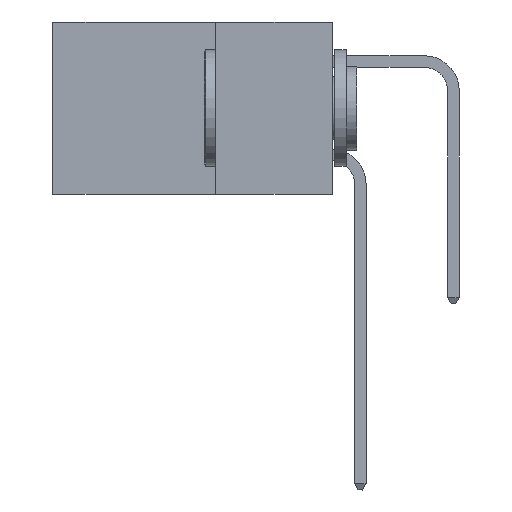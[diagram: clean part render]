
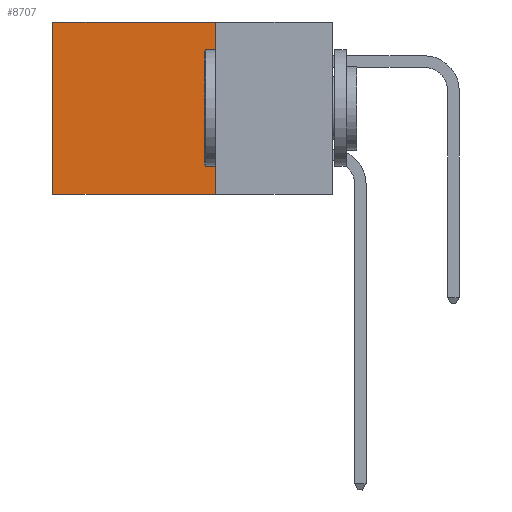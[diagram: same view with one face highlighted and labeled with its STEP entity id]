
A CAD part, left-side view. The second image highlights one B-rep face of the part: STEP entity #8707.
In plain terms, the highlighted planar face has unit normal (-1, 0, 0).
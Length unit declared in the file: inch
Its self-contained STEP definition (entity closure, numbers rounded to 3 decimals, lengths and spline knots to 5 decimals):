
#2173 = VERTEX_POINT ( 'NONE', #23005 ) ;
#2880 = LINE ( 'NONE', #3835, #20670 ) ;
#3231 = VERTEX_POINT ( 'NONE', #19657 ) ;
#3835 = CARTESIAN_POINT ( 'NONE',  ( 0.298, 0.25, 0. ) ) ;
#6220 = DIRECTION ( 'NONE',  ( 0., 0., -1. ) ) ;
#6695 = VECTOR ( 'NONE', #28479, 39.37008 ) ;
#6897 = CARTESIAN_POINT ( 'NONE',  ( 0.298, 0.6, -0.37 ) ) ;
#7433 = LINE ( 'NONE', #26157, #6695 ) ;
#7675 = ORIENTED_EDGE ( 'NONE', *, *, #19054, .T. ) ;
#8707 = ADVANCED_FACE ( 'NONE', ( #20876 ), #25672, .F. ) ;
#11441 = CARTESIAN_POINT ( 'NONE',  ( 0.298, 0.25, 0. ) ) ;
#13474 = EDGE_CURVE ( 'NONE', #2173, #17907, #7433, .T. ) ;
#13802 = DIRECTION ( 'NONE',  ( 0., 0., -1. ) ) ;
#14105 = EDGE_LOOP ( 'NONE', ( #31052, #15965, #26551, #7675 ) ) ;
#15561 = VECTOR ( 'NONE', #30053, 39.37008 ) ;
#15965 = ORIENTED_EDGE ( 'NONE', *, *, #29379, .F. ) ;
#15981 = VECTOR ( 'NONE', #29298, 39.37008 ) ;
#17104 = LINE ( 'NONE', #27704, #15561 ) ;
#17907 = VERTEX_POINT ( 'NONE', #6897 ) ;
#19054 = EDGE_CURVE ( 'NONE', #25901, #2173, #17104, .T. ) ;
#19400 = CARTESIAN_POINT ( 'NONE',  ( 0.298, 0.25, -0.37 ) ) ;
#19657 = CARTESIAN_POINT ( 'NONE',  ( 0.298, 0.25, -0.37 ) ) ;
#19783 = CARTESIAN_POINT ( 'NONE',  ( 0.298, 0.25, 0. ) ) ;
#20670 = VECTOR ( 'NONE', #6220, 39.37008 ) ;
#20876 = FACE_OUTER_BOUND ( 'NONE', #14105, .T. ) ;
#23005 = CARTESIAN_POINT ( 'NONE',  ( 0.298, 0.6, 0. ) ) ;
#23292 = AXIS2_PLACEMENT_3D ( 'NONE', #11441, #28088, #13802 ) ;
#24296 = EDGE_CURVE ( 'NONE', #25901, #3231, #2880, .T. ) ;
#25672 = PLANE ( 'NONE',  #23292 ) ;
#25901 = VERTEX_POINT ( 'NONE', #19783 ) ;
#26157 = CARTESIAN_POINT ( 'NONE',  ( 0.298, 0.6, 0. ) ) ;
#26551 = ORIENTED_EDGE ( 'NONE', *, *, #24296, .F. ) ;
#27704 = CARTESIAN_POINT ( 'NONE',  ( 0.298, 0.25, 0. ) ) ;
#28088 = DIRECTION ( 'NONE',  ( 1., 0., 0. ) ) ;
#28479 = DIRECTION ( 'NONE',  ( 0., 0., -1. ) ) ;
#28627 = LINE ( 'NONE', #19400, #15981 ) ;
#29298 = DIRECTION ( 'NONE',  ( 0., 1., 0. ) ) ;
#29379 = EDGE_CURVE ( 'NONE', #3231, #17907, #28627, .T. ) ;
#30053 = DIRECTION ( 'NONE',  ( 0., 1., 0. ) ) ;
#31052 = ORIENTED_EDGE ( 'NONE', *, *, #13474, .T. ) ;
